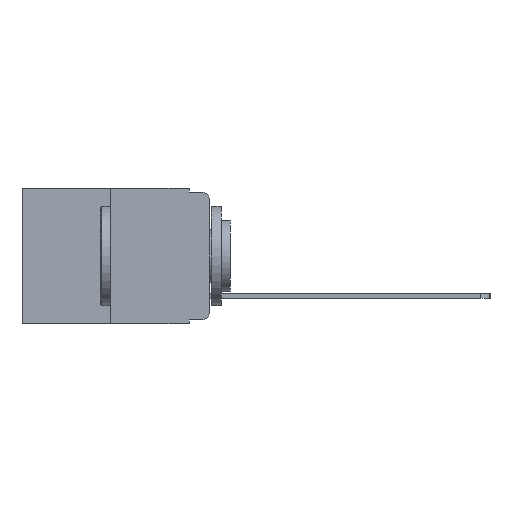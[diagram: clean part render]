
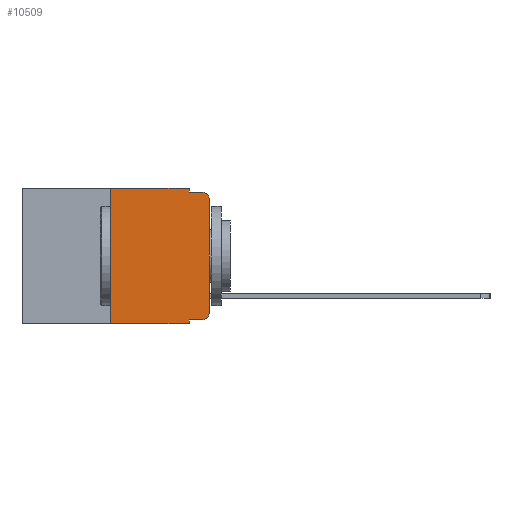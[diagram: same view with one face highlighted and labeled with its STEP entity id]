
A CAD part, left-side view. The second image highlights one B-rep face of the part: STEP entity #10509.
In plain terms, the highlighted planar face has unit normal (-1, 0, 0).
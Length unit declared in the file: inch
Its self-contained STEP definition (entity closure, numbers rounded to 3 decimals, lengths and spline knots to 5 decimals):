
#30 = CARTESIAN_POINT ( 'NONE',  ( 0., 0., 0. ) ) ;
#90 = VECTOR ( 'NONE', #14163, 39.37008 ) ;
#992 = VECTOR ( 'NONE', #21080, 39.37008 ) ;
#1310 = EDGE_CURVE ( 'NONE', #7934, #13145, #4448, .T. ) ;
#1336 = VERTEX_POINT ( 'NONE', #9298 ) ;
#1604 = EDGE_CURVE ( 'NONE', #12060, #11692, #9630, .T. ) ;
#1793 = VECTOR ( 'NONE', #7149, 39.37008 ) ;
#2079 = CIRCLE ( 'NONE', #10824, 0.02 ) ;
#2438 = DIRECTION ( 'NONE',  ( 0., 0., 1. ) ) ;
#2590 = EDGE_CURVE ( 'NONE', #13145, #10759, #2079, .T. ) ;
#2844 = ORIENTED_EDGE ( 'NONE', *, *, #2590, .T. ) ;
#3294 = CARTESIAN_POINT ( 'NONE',  ( 0., 0.02, -0.313 ) ) ;
#3304 = VERTEX_POINT ( 'NONE', #14283 ) ;
#3841 = VECTOR ( 'NONE', #4331, 39.37008 ) ;
#4252 = CARTESIAN_POINT ( 'NONE',  ( 0., 0., -0.03 ) ) ;
#4331 = DIRECTION ( 'NONE',  ( 0., -1., 0. ) ) ;
#4385 = EDGE_LOOP ( 'NONE', ( #16017, #2844, #13694, #10278, #15245, #6982, #20822, #4510, #9710, #14714 ) ) ;
#4448 = LINE ( 'NONE', #30, #8579 ) ;
#4510 = ORIENTED_EDGE ( 'NONE', *, *, #7626, .F. ) ;
#4666 = CARTESIAN_POINT ( 'NONE',  ( 0., 0.051, -0.343 ) ) ;
#5097 = DIRECTION ( 'NONE',  ( 0., 0., -1. ) ) ;
#5401 = CARTESIAN_POINT ( 'NONE',  ( 0., 0.051, -0.01 ) ) ;
#5623 = PLANE ( 'NONE',  #15834 ) ;
#5632 = CARTESIAN_POINT ( 'NONE',  ( 0., 0.473, 0. ) ) ;
#6377 = LINE ( 'NONE', #7708, #14890 ) ;
#6982 = ORIENTED_EDGE ( 'NONE', *, *, #1604, .F. ) ;
#7129 = LINE ( 'NONE', #5401, #1793 ) ;
#7149 = DIRECTION ( 'NONE',  ( 0., -1., 0. ) ) ;
#7444 = DIRECTION ( 'NONE',  ( 0., 0., -1. ) ) ;
#7502 = VERTEX_POINT ( 'NONE', #12424 ) ;
#7537 = DIRECTION ( 'NONE',  ( 0., 0., 1. ) ) ;
#7626 = EDGE_CURVE ( 'NONE', #7502, #22035, #6377, .T. ) ;
#7708 = CARTESIAN_POINT ( 'NONE',  ( 0., 0.051, 0. ) ) ;
#7720 = CARTESIAN_POINT ( 'NONE',  ( 0., 0.25, 0. ) ) ;
#7934 = VERTEX_POINT ( 'NONE', #20166 ) ;
#8420 = LINE ( 'NONE', #15390, #11365 ) ;
#8533 = LINE ( 'NONE', #17990, #3841 ) ;
#8579 = VECTOR ( 'NONE', #2438, 39.37008 ) ;
#8612 = FACE_OUTER_BOUND ( 'NONE', #4385, .T. ) ;
#8814 = DIRECTION ( 'NONE',  ( -1., 0., 0. ) ) ;
#9298 = CARTESIAN_POINT ( 'NONE',  ( 0., 0.051, -0.01 ) ) ;
#9498 = CARTESIAN_POINT ( 'NONE',  ( 0., 0.051, 0. ) ) ;
#9630 = LINE ( 'NONE', #7720, #18041 ) ;
#9710 = ORIENTED_EDGE ( 'NONE', *, *, #15520, .T. ) ;
#10278 = ORIENTED_EDGE ( 'NONE', *, *, #10662, .F. ) ;
#10509 = ADVANCED_FACE ( 'NONE', ( #8612 ), #5623, .F. ) ;
#10662 = EDGE_CURVE ( 'NONE', #3304, #1336, #19317, .T. ) ;
#10759 = VERTEX_POINT ( 'NONE', #18163 ) ;
#10824 = AXIS2_PLACEMENT_3D ( 'NONE', #14058, #8814, #14447 ) ;
#11271 = LINE ( 'NONE', #5632, #90 ) ;
#11365 = VECTOR ( 'NONE', #17087, 39.37008 ) ;
#11381 = CARTESIAN_POINT ( 'NONE',  ( 0., 0.25, 0. ) ) ;
#11394 = EDGE_CURVE ( 'NONE', #11692, #3304, #11271, .T. ) ;
#11692 = VERTEX_POINT ( 'NONE', #11381 ) ;
#12060 = VERTEX_POINT ( 'NONE', #22090 ) ;
#12264 = AXIS2_PLACEMENT_3D ( 'NONE', #3294, #15314, #5097 ) ;
#12424 = CARTESIAN_POINT ( 'NONE',  ( 0., 0.051, -0.333 ) ) ;
#13145 = VERTEX_POINT ( 'NONE', #4252 ) ;
#13452 = EDGE_CURVE ( 'NONE', #19739, #7934, #18260, .T. ) ;
#13642 = EDGE_CURVE ( 'NONE', #1336, #10759, #7129, .T. ) ;
#13694 = ORIENTED_EDGE ( 'NONE', *, *, #13642, .F. ) ;
#14058 = CARTESIAN_POINT ( 'NONE',  ( 0., 0.02, -0.03 ) ) ;
#14163 = DIRECTION ( 'NONE',  ( 0., -1., 0. ) ) ;
#14226 = CARTESIAN_POINT ( 'NONE',  ( 0., 0.473, 0. ) ) ;
#14283 = CARTESIAN_POINT ( 'NONE',  ( 0., 0.051, 0. ) ) ;
#14447 = DIRECTION ( 'NONE',  ( 0., 0., -1. ) ) ;
#14714 = ORIENTED_EDGE ( 'NONE', *, *, #13452, .T. ) ;
#14890 = VECTOR ( 'NONE', #19409, 39.37008 ) ;
#15245 = ORIENTED_EDGE ( 'NONE', *, *, #11394, .F. ) ;
#15314 = DIRECTION ( 'NONE',  ( -1., 0., 0. ) ) ;
#15390 = CARTESIAN_POINT ( 'NONE',  ( 0., 0.473, -0.343 ) ) ;
#15520 = EDGE_CURVE ( 'NONE', #7502, #19739, #8533, .T. ) ;
#15834 = AXIS2_PLACEMENT_3D ( 'NONE', #14226, #17572, #7444 ) ;
#16017 = ORIENTED_EDGE ( 'NONE', *, *, #1310, .T. ) ;
#16284 = CARTESIAN_POINT ( 'NONE',  ( 0., 0.02, -0.333 ) ) ;
#17087 = DIRECTION ( 'NONE',  ( 0., -1., 0. ) ) ;
#17572 = DIRECTION ( 'NONE',  ( 1., 0., 0. ) ) ;
#17990 = CARTESIAN_POINT ( 'NONE',  ( 0., 0.051, -0.333 ) ) ;
#18041 = VECTOR ( 'NONE', #7537, 39.37008 ) ;
#18163 = CARTESIAN_POINT ( 'NONE',  ( 0., 0.02, -0.01 ) ) ;
#18260 = CIRCLE ( 'NONE', #12264, 0.02 ) ;
#19317 = LINE ( 'NONE', #9498, #992 ) ;
#19409 = DIRECTION ( 'NONE',  ( 0., 0., -1. ) ) ;
#19739 = VERTEX_POINT ( 'NONE', #16284 ) ;
#20166 = CARTESIAN_POINT ( 'NONE',  ( 0., 0., -0.313 ) ) ;
#20791 = EDGE_CURVE ( 'NONE', #12060, #22035, #8420, .T. ) ;
#20822 = ORIENTED_EDGE ( 'NONE', *, *, #20791, .T. ) ;
#21080 = DIRECTION ( 'NONE',  ( 0., 0., -1. ) ) ;
#22035 = VERTEX_POINT ( 'NONE', #4666 ) ;
#22090 = CARTESIAN_POINT ( 'NONE',  ( 0., 0.25, -0.343 ) ) ;
